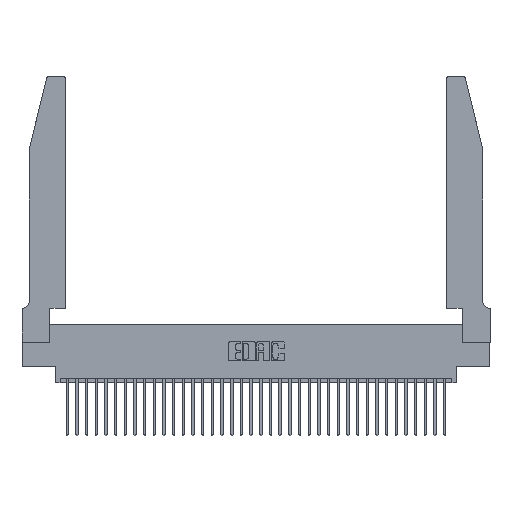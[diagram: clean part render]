
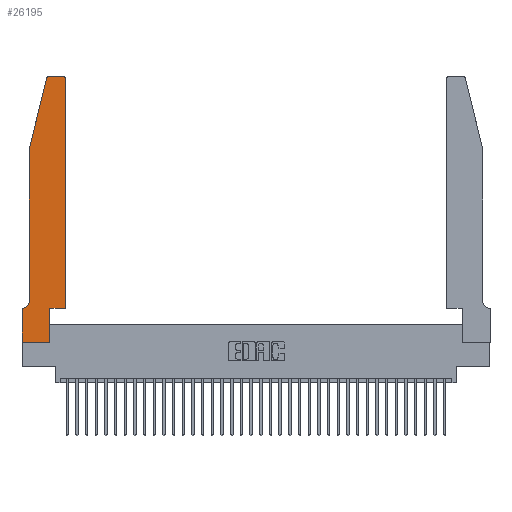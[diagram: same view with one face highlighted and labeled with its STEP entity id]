
A CAD part, top view. The second image highlights one B-rep face of the part: STEP entity #26195.
In plain terms, the highlighted planar face has unit normal (0, 0, 1).
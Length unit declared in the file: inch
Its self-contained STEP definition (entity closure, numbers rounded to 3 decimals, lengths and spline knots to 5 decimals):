
#36 = EDGE_CURVE ( 'NONE', #32635, #30305, #19986, .T. ) ;
#109 = CARTESIAN_POINT ( 'NONE',  ( 0.4505, 0.35, 0.37 ) ) ;
#550 = CIRCLE ( 'NONE', #7999, 0.03 ) ;
#1394 = EDGE_CURVE ( 'NONE', #22809, #30964, #9078, .T. ) ;
#1422 = CARTESIAN_POINT ( 'NONE',  ( 0.4505, 0.35, 0.37 ) ) ;
#1732 = LINE ( 'NONE', #1422, #17704 ) ;
#2122 = AXIS2_PLACEMENT_3D ( 'NONE', #6282, #31761, #34588 ) ;
#2340 = CARTESIAN_POINT ( 'NONE',  ( 0.284, 2.75, 0.37 ) ) ;
#2899 = CARTESIAN_POINT ( 'NONE',  ( 0.0055, 0.35, 0.37 ) ) ;
#3216 = DIRECTION ( 'NONE',  ( 0., 0., 1. ) ) ;
#3622 = LINE ( 'NONE', #16483, #16987 ) ;
#4135 = CARTESIAN_POINT ( 'NONE',  ( 0., 0., 0.37 ) ) ;
#4659 = CARTESIAN_POINT ( 'NONE',  ( 0., 0., 0.37 ) ) ;
#5436 = EDGE_CURVE ( 'NONE', #12074, #8704, #7537, .T. ) ;
#6136 = CARTESIAN_POINT ( 'NONE',  ( 0.4505, 0.35, 0.37 ) ) ;
#6282 = CARTESIAN_POINT ( 'NONE',  ( 0., 0.35, 0.37 ) ) ;
#6481 = DIRECTION ( 'NONE',  ( 0., -1., 0. ) ) ;
#6516 = CARTESIAN_POINT ( 'NONE',  ( 0.0755, 2., 0.37 ) ) ;
#6765 = ORIENTED_EDGE ( 'NONE', *, *, #29344, .T. ) ;
#7217 = VERTEX_POINT ( 'NONE', #10940 ) ;
#7232 = VERTEX_POINT ( 'NONE', #2340 ) ;
#7537 = LINE ( 'NONE', #109, #29097 ) ;
#7627 = ORIENTED_EDGE ( 'NONE', *, *, #32203, .T. ) ;
#7999 = AXIS2_PLACEMENT_3D ( 'NONE', #36445, #27995, #30912 ) ;
#8337 = LINE ( 'NONE', #35616, #30300 ) ;
#8486 = CARTESIAN_POINT ( 'NONE',  ( 0.2605, 2.75, 0.37 ) ) ;
#8632 = ORIENTED_EDGE ( 'NONE', *, *, #36, .T. ) ;
#8704 = VERTEX_POINT ( 'NONE', #14863 ) ;
#9078 = CIRCLE ( 'NONE', #20640, 0.07 ) ;
#9284 = VECTOR ( 'NONE', #12448, 39.37008 ) ;
#9378 = VECTOR ( 'NONE', #35456, 39.37008 ) ;
#9682 = CARTESIAN_POINT ( 'NONE',  ( 0.0755, 0.35, 0.37 ) ) ;
#9905 = EDGE_CURVE ( 'NONE', #30305, #24624, #8337, .T. ) ;
#10221 = CARTESIAN_POINT ( 'NONE',  ( 0.0055, 0.42, 0.37 ) ) ;
#10940 = CARTESIAN_POINT ( 'NONE',  ( 0.4205, 2.75, 0.37 ) ) ;
#12012 = VERTEX_POINT ( 'NONE', #33324 ) ;
#12074 = VERTEX_POINT ( 'NONE', #6136 ) ;
#12448 = DIRECTION ( 'NONE',  ( -0.239, -0.971, 0. ) ) ;
#13148 = DIRECTION ( 'NONE',  ( -1., 0., 0. ) ) ;
#13973 = VERTEX_POINT ( 'NONE', #29642 ) ;
#14863 = CARTESIAN_POINT ( 'NONE',  ( 0.4505, 2.72, 0.37 ) ) ;
#15954 = ORIENTED_EDGE ( 'NONE', *, *, #1394, .T. ) ;
#16000 = FACE_OUTER_BOUND ( 'NONE', #36251, .T. ) ;
#16483 = CARTESIAN_POINT ( 'NONE',  ( 0.0755, 2., 0.37 ) ) ;
#16492 = EDGE_CURVE ( 'NONE', #8704, #7217, #550, .T. ) ;
#16928 = VERTEX_POINT ( 'NONE', #24886 ) ;
#16987 = VECTOR ( 'NONE', #36172, 39.37008 ) ;
#17704 = VECTOR ( 'NONE', #20993, 39.37008 ) ;
#18079 = CARTESIAN_POINT ( 'NONE',  ( 0., 0., 0.37 ) ) ;
#18089 = VECTOR ( 'NONE', #6481, 39.37008 ) ;
#18365 = ORIENTED_EDGE ( 'NONE', *, *, #18954, .T. ) ;
#18954 = EDGE_CURVE ( 'NONE', #24624, #12074, #1732, .T. ) ;
#19630 = ORIENTED_EDGE ( 'NONE', *, *, #9905, .T. ) ;
#19934 = DIRECTION ( 'NONE',  ( 0., 1., 0. ) ) ;
#19986 = LINE ( 'NONE', #4659, #9378 ) ;
#20434 = EDGE_CURVE ( 'NONE', #7232, #16928, #25625, .T. ) ;
#20640 = AXIS2_PLACEMENT_3D ( 'NONE', #10221, #35551, #13148 ) ;
#20698 = EDGE_CURVE ( 'NONE', #16928, #13973, #25678, .T. ) ;
#20703 = EDGE_CURVE ( 'NONE', #12012, #32635, #24310, .T. ) ;
#20814 = LINE ( 'NONE', #9682, #30143 ) ;
#20973 = DIRECTION ( 'NONE',  ( -1., 0., 0. ) ) ;
#20993 = DIRECTION ( 'NONE',  ( 1., 0., 0. ) ) ;
#21188 = DIRECTION ( 'NONE',  ( 0., 1., 0. ) ) ;
#21395 = CARTESIAN_POINT ( 'NONE',  ( 0.2865, 0.35, 0.37 ) ) ;
#22151 = CARTESIAN_POINT ( 'NONE',  ( 0.0755, 0.42, 0.37 ) ) ;
#22809 = VERTEX_POINT ( 'NONE', #22151 ) ;
#22985 = PLANE ( 'NONE',  #2122 ) ;
#23802 = VECTOR ( 'NONE', #28188, 39.37008 ) ;
#24296 = AXIS2_PLACEMENT_3D ( 'NONE', #27993, #3216, #25403 ) ;
#24310 = LINE ( 'NONE', #4135, #18089 ) ;
#24624 = VERTEX_POINT ( 'NONE', #21395 ) ;
#24886 = CARTESIAN_POINT ( 'NONE',  ( 0.25487, 2.72718, 0.37 ) ) ;
#25403 = DIRECTION ( 'NONE',  ( 1., 0., 0. ) ) ;
#25625 = CIRCLE ( 'NONE', #24296, 0.03 ) ;
#25678 = LINE ( 'NONE', #6516, #9284 ) ;
#26195 = ADVANCED_FACE ( 'NONE', ( #16000 ), #22985, .T. ) ;
#26337 = ORIENTED_EDGE ( 'NONE', *, *, #20703, .T. ) ;
#27993 = CARTESIAN_POINT ( 'NONE',  ( 0.284, 2.72, 0.37 ) ) ;
#27995 = DIRECTION ( 'NONE',  ( 0., 0., 1. ) ) ;
#28108 = LINE ( 'NONE', #8486, #23802 ) ;
#28188 = DIRECTION ( 'NONE',  ( -1., 0., 0. ) ) ;
#28427 = CARTESIAN_POINT ( 'NONE',  ( 0.2865, 0., 0.37 ) ) ;
#28706 = EDGE_CURVE ( 'NONE', #13973, #22809, #3622, .T. ) ;
#29097 = VECTOR ( 'NONE', #19934, 39.37008 ) ;
#29344 = EDGE_CURVE ( 'NONE', #30964, #12012, #20814, .T. ) ;
#29642 = CARTESIAN_POINT ( 'NONE',  ( 0.0755, 2., 0.37 ) ) ;
#29728 = ORIENTED_EDGE ( 'NONE', *, *, #20434, .T. ) ;
#30143 = VECTOR ( 'NONE', #20973, 39.37008 ) ;
#30300 = VECTOR ( 'NONE', #21188, 39.37008 ) ;
#30305 = VERTEX_POINT ( 'NONE', #28427 ) ;
#30912 = DIRECTION ( 'NONE',  ( 1., 0., 0. ) ) ;
#30947 = ORIENTED_EDGE ( 'NONE', *, *, #16492, .T. ) ;
#30964 = VERTEX_POINT ( 'NONE', #2899 ) ;
#31761 = DIRECTION ( 'NONE',  ( 0., 0., 1. ) ) ;
#31941 = ORIENTED_EDGE ( 'NONE', *, *, #20698, .T. ) ;
#32203 = EDGE_CURVE ( 'NONE', #7217, #7232, #28108, .T. ) ;
#32635 = VERTEX_POINT ( 'NONE', #18079 ) ;
#33324 = CARTESIAN_POINT ( 'NONE',  ( 0., 0.35, 0.37 ) ) ;
#34227 = ORIENTED_EDGE ( 'NONE', *, *, #28706, .T. ) ;
#34588 = DIRECTION ( 'NONE',  ( 1., 0., 0. ) ) ;
#35456 = DIRECTION ( 'NONE',  ( 1., 0., 0. ) ) ;
#35551 = DIRECTION ( 'NONE',  ( 0., 0., -1. ) ) ;
#35616 = CARTESIAN_POINT ( 'NONE',  ( 0.2865, 0.35, 0.37 ) ) ;
#35697 = ORIENTED_EDGE ( 'NONE', *, *, #5436, .T. ) ;
#36172 = DIRECTION ( 'NONE',  ( 0., -1., 0. ) ) ;
#36251 = EDGE_LOOP ( 'NONE', ( #7627, #29728, #31941, #34227, #15954, #6765, #26337, #8632, #19630, #18365, #35697, #30947 ) ) ;
#36445 = CARTESIAN_POINT ( 'NONE',  ( 0.4205, 2.72, 0.37 ) ) ;
